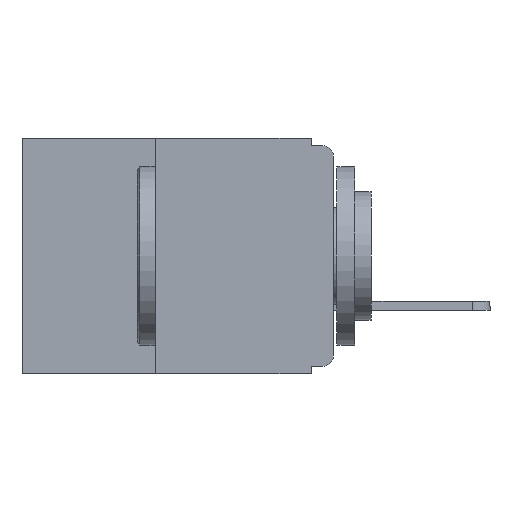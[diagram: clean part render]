
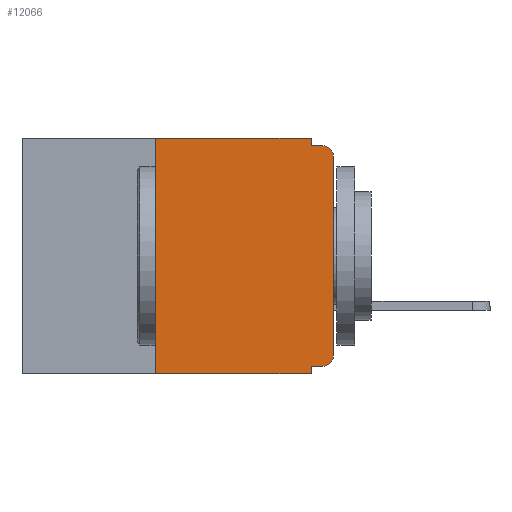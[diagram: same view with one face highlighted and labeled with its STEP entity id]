
A CAD part, left-side view. The second image highlights one B-rep face of the part: STEP entity #12066.
In plain terms, the highlighted planar face has unit normal (-1, 0, 0).
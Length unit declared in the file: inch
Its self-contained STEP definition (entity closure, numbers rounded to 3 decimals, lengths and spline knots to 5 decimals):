
#3 = LINE ( 'NONE', #6223, #18694 ) ;
#43 = CARTESIAN_POINT ( 'NONE',  ( 0., 0., -0.025 ) ) ;
#161 = DIRECTION ( 'NONE',  ( -1., 0., 0. ) ) ;
#242 = LINE ( 'NONE', #21719, #8764 ) ;
#267 = EDGE_CURVE ( 'NONE', #22800, #20154, #3, .T. ) ;
#506 = VECTOR ( 'NONE', #4750, 39.37008 ) ;
#608 = DIRECTION ( 'NONE',  ( 0., 0., -1. ) ) ;
#898 = VECTOR ( 'NONE', #6030, 39.37008 ) ;
#1059 = LINE ( 'NONE', #13771, #506 ) ;
#1459 = DIRECTION ( 'NONE',  ( -1., 0., 0. ) ) ;
#1507 = DIRECTION ( 'NONE',  ( 0., 0., 1. ) ) ;
#2201 = LINE ( 'NONE', #7037, #7649 ) ;
#2252 = AXIS2_PLACEMENT_3D ( 'NONE', #2374, #11467, #608 ) ;
#2374 = CARTESIAN_POINT ( 'NONE',  ( 0., 0.437, 0. ) ) ;
#3679 = CARTESIAN_POINT ( 'NONE',  ( 0., 0.015, -0.01 ) ) ;
#3781 = DIRECTION ( 'NONE',  ( 0., 0., 1. ) ) ;
#4268 = ORIENTED_EDGE ( 'NONE', *, *, #19917, .T. ) ;
#4356 = VECTOR ( 'NONE', #5020, 39.37008 ) ;
#4750 = DIRECTION ( 'NONE',  ( 0., -1., 0. ) ) ;
#5020 = DIRECTION ( 'NONE',  ( 0., 1., 0. ) ) ;
#5361 = ORIENTED_EDGE ( 'NONE', *, *, #20787, .F. ) ;
#5641 = EDGE_CURVE ( 'NONE', #13647, #22800, #8596, .T. ) ;
#5812 = VERTEX_POINT ( 'NONE', #43 ) ;
#5876 = VECTOR ( 'NONE', #15628, 39.37008 ) ;
#5922 = CIRCLE ( 'NONE', #12985, 0.015 ) ;
#6025 = VERTEX_POINT ( 'NONE', #22210 ) ;
#6030 = DIRECTION ( 'NONE',  ( 0., -1., 0. ) ) ;
#6223 = CARTESIAN_POINT ( 'NONE',  ( 0., 0.031, -0.33 ) ) ;
#6296 = EDGE_CURVE ( 'NONE', #5812, #13107, #16774, .T. ) ;
#6865 = CARTESIAN_POINT ( 'NONE',  ( 0., 0., -0.32 ) ) ;
#7037 = CARTESIAN_POINT ( 'NONE',  ( 0., 0.25, -0.33 ) ) ;
#7649 = VECTOR ( 'NONE', #1507, 39.37008 ) ;
#7898 = VERTEX_POINT ( 'NONE', #20836 ) ;
#7930 = ORIENTED_EDGE ( 'NONE', *, *, #14598, .F. ) ;
#8038 = ORIENTED_EDGE ( 'NONE', *, *, #8526, .F. ) ;
#8215 = ORIENTED_EDGE ( 'NONE', *, *, #267, .F. ) ;
#8526 = EDGE_CURVE ( 'NONE', #14083, #13107, #1059, .T. ) ;
#8596 = LINE ( 'NONE', #6865, #4356 ) ;
#8764 = VECTOR ( 'NONE', #3781, 39.37008 ) ;
#9080 = CARTESIAN_POINT ( 'NONE',  ( 0., 0.031, -0.33 ) ) ;
#9342 = EDGE_CURVE ( 'NONE', #13647, #6025, #5922, .T. ) ;
#9439 = CARTESIAN_POINT ( 'NONE',  ( 0., 0.25, -0.33 ) ) ;
#10258 = ORIENTED_EDGE ( 'NONE', *, *, #16872, .T. ) ;
#10550 = LINE ( 'NONE', #11351, #898 ) ;
#10794 = EDGE_LOOP ( 'NONE', ( #10258, #15379, #8038, #5361, #7930, #22615, #4268, #8215, #12170, #11323 ) ) ;
#10942 = DIRECTION ( 'NONE',  ( 0., 0., -1. ) ) ;
#11035 = CARTESIAN_POINT ( 'NONE',  ( 0., 0.015, -0.305 ) ) ;
#11323 = ORIENTED_EDGE ( 'NONE', *, *, #9342, .T. ) ;
#11351 = CARTESIAN_POINT ( 'NONE',  ( 0., 0.437, 0. ) ) ;
#11467 = DIRECTION ( 'NONE',  ( 1., 0., 0. ) ) ;
#12030 = CARTESIAN_POINT ( 'NONE',  ( 0., 0.25, 0. ) ) ;
#12066 = ADVANCED_FACE ( 'NONE', ( #14922 ), #22212, .F. ) ;
#12170 = ORIENTED_EDGE ( 'NONE', *, *, #5641, .F. ) ;
#12339 = CARTESIAN_POINT ( 'NONE',  ( 0., 0.015, -0.025 ) ) ;
#12881 = DIRECTION ( 'NONE',  ( 0., 0., -1. ) ) ;
#12985 = AXIS2_PLACEMENT_3D ( 'NONE', #11035, #161, #12881 ) ;
#13107 = VERTEX_POINT ( 'NONE', #3679 ) ;
#13244 = VERTEX_POINT ( 'NONE', #9439 ) ;
#13647 = VERTEX_POINT ( 'NONE', #15877 ) ;
#13771 = CARTESIAN_POINT ( 'NONE',  ( 0., 0., -0.01 ) ) ;
#14083 = VERTEX_POINT ( 'NONE', #15231 ) ;
#14164 = DIRECTION ( 'NONE',  ( 0., 0., -1. ) ) ;
#14287 = VECTOR ( 'NONE', #10942, 39.37008 ) ;
#14525 = CARTESIAN_POINT ( 'NONE',  ( 0., 0.031, 0. ) ) ;
#14598 = EDGE_CURVE ( 'NONE', #19914, #7898, #10550, .T. ) ;
#14922 = FACE_OUTER_BOUND ( 'NONE', #10794, .T. ) ;
#15231 = CARTESIAN_POINT ( 'NONE',  ( 0., 0.031, -0.01 ) ) ;
#15379 = ORIENTED_EDGE ( 'NONE', *, *, #6296, .T. ) ;
#15628 = DIRECTION ( 'NONE',  ( 0., -1., 0. ) ) ;
#15877 = CARTESIAN_POINT ( 'NONE',  ( 0., 0.015, -0.32 ) ) ;
#16774 = CIRCLE ( 'NONE', #20277, 0.015 ) ;
#16872 = EDGE_CURVE ( 'NONE', #6025, #5812, #242, .T. ) ;
#17362 = EDGE_CURVE ( 'NONE', #13244, #19914, #2201, .T. ) ;
#18694 = VECTOR ( 'NONE', #22184, 39.37008 ) ;
#19047 = LINE ( 'NONE', #14525, #14287 ) ;
#19311 = CARTESIAN_POINT ( 'NONE',  ( 0., 0.031, -0.32 ) ) ;
#19914 = VERTEX_POINT ( 'NONE', #12030 ) ;
#19917 = EDGE_CURVE ( 'NONE', #13244, #20154, #20181, .T. ) ;
#20154 = VERTEX_POINT ( 'NONE', #9080 ) ;
#20181 = LINE ( 'NONE', #22732, #5876 ) ;
#20277 = AXIS2_PLACEMENT_3D ( 'NONE', #12339, #1459, #14164 ) ;
#20787 = EDGE_CURVE ( 'NONE', #7898, #14083, #19047, .T. ) ;
#20836 = CARTESIAN_POINT ( 'NONE',  ( 0., 0.031, 0. ) ) ;
#21719 = CARTESIAN_POINT ( 'NONE',  ( 0., 0., 0. ) ) ;
#22184 = DIRECTION ( 'NONE',  ( 0., 0., -1. ) ) ;
#22210 = CARTESIAN_POINT ( 'NONE',  ( 0., 0., -0.305 ) ) ;
#22212 = PLANE ( 'NONE',  #2252 ) ;
#22615 = ORIENTED_EDGE ( 'NONE', *, *, #17362, .F. ) ;
#22732 = CARTESIAN_POINT ( 'NONE',  ( 0., 0.437, -0.33 ) ) ;
#22800 = VERTEX_POINT ( 'NONE', #19311 ) ;
